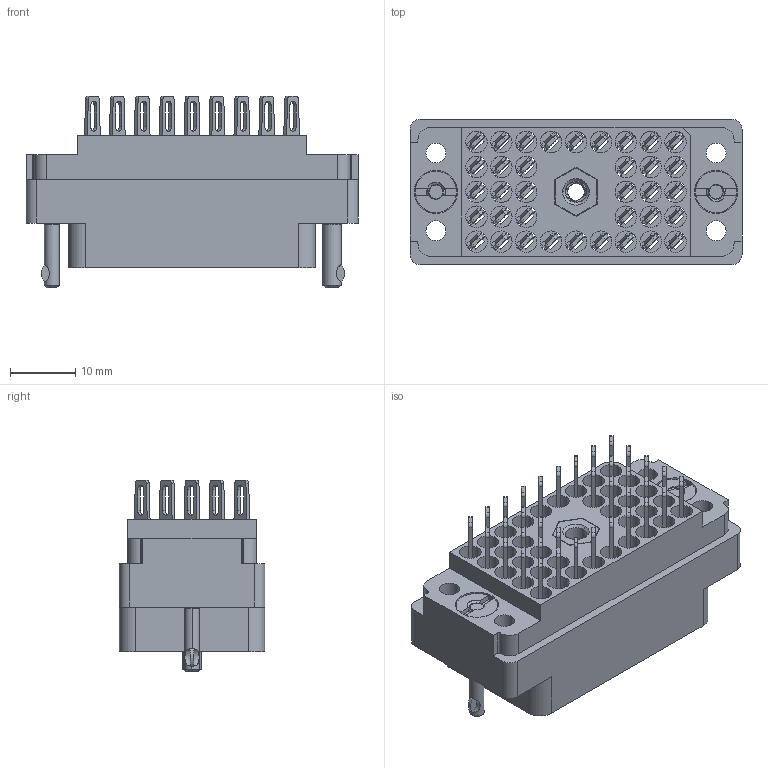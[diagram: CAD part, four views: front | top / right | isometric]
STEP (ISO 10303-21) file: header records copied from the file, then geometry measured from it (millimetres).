
FILE_DESCRIPTION (( 'STEP AP203' ), '1' );
FILE_NAME ('519-036-500-302.STEP', '2020-03-11T16:07:06', ( '' ), ( '' ), 'SwSTEP 2.0', 'SolidWorks 2016', '' );
FILE_SCHEMA (( 'CONFIG_CONTROL_DESIGN' ));
Length unit declared in the file: inch
Products named in the file (7): 516-222-038-102_039; 519-036-500-302; 516-222-038-102_038; 516-252-021-102_038; 516-252-035-100_516-252-035-100; 519 Plug Insulator_036; 516-292-001_500 Contact
Assembly tree (42 placements, depth 2):
  519-036-500-302
    519 Plug Insulator_036
    516-292-001_500 Contact  x36
    516-252-035-100_516-252-035-100
    516-252-021-102_038  x2
    516-222-038-102_038
    516-222-038-102_039
Bounding box: 50.8 x 22.25 x 29.36 mm (x, y, z)
Volume: 10859.3 mm3; surface area: 19061.8 mm2
Topology: 42 solids, 42 shells, 3828 faces, 11031 edges, 7310 vertices
Faces by surface type: plane 2218, cylinder 1302, bspline 258, cone 46, torus 4
Entity records: 45814 total; most frequent: CARTESIAN_POINT 14095, ORIENTED_EDGE 6482, DIRECTION 6081, EDGE_CURVE 3241, VECTOR 2169, LINE 2169, VERTEX_POINT 2140, AXIS2_PLACEMENT_3D 1956
